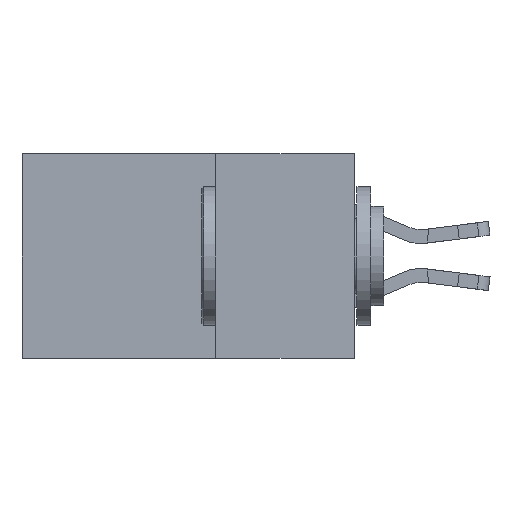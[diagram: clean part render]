
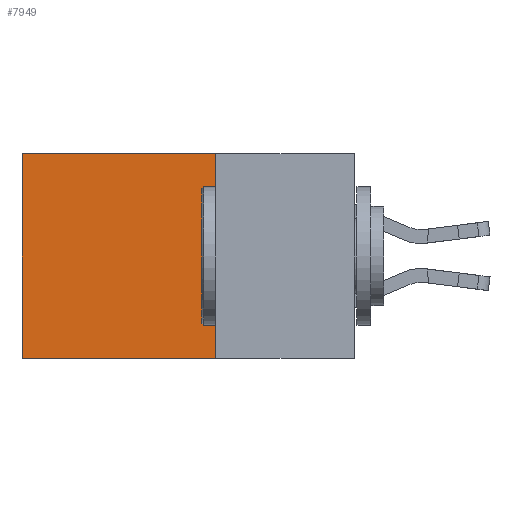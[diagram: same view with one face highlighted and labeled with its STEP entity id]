
A CAD part, left-side view. The second image highlights one B-rep face of the part: STEP entity #7949.
In plain terms, the highlighted planar face has unit normal (-1, 0, 0).
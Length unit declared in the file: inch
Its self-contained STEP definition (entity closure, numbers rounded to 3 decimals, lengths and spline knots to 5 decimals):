
#158 = DIRECTION ( 'NONE',  ( 0., 1., 0. ) ) ;
#1003 = EDGE_CURVE ( 'NONE', #11231, #4070, #4851, .T. ) ;
#1647 = ORIENTED_EDGE ( 'NONE', *, *, #11273, .F. ) ;
#1665 = VECTOR ( 'NONE', #3794, 39.37008 ) ;
#2700 = VERTEX_POINT ( 'NONE', #12612 ) ;
#3143 = VERTEX_POINT ( 'NONE', #5457 ) ;
#3479 = CARTESIAN_POINT ( 'NONE',  ( 0.2615, 0.25, -0.37 ) ) ;
#3794 = DIRECTION ( 'NONE',  ( 0., 1., 0. ) ) ;
#3870 = CARTESIAN_POINT ( 'NONE',  ( 0.2615, 0.25, 0. ) ) ;
#4070 = VERTEX_POINT ( 'NONE', #4142 ) ;
#4142 = CARTESIAN_POINT ( 'NONE',  ( 0.2615, 0.6, -0.37 ) ) ;
#4332 = LINE ( 'NONE', #3870, #1665 ) ;
#4844 = FACE_OUTER_BOUND ( 'NONE', #11598, .T. ) ;
#4851 = LINE ( 'NONE', #7050, #14524 ) ;
#4900 = CARTESIAN_POINT ( 'NONE',  ( 0.2615, 0.6, 0. ) ) ;
#5062 = DIRECTION ( 'NONE',  ( 0., 0., -1. ) ) ;
#5071 = AXIS2_PLACEMENT_3D ( 'NONE', #7172, #6859, #6843 ) ;
#5457 = CARTESIAN_POINT ( 'NONE',  ( 0.2615, 0.25, 0. ) ) ;
#6830 = VECTOR ( 'NONE', #5062, 39.37008 ) ;
#6843 = DIRECTION ( 'NONE',  ( 0., 0., -1. ) ) ;
#6859 = DIRECTION ( 'NONE',  ( 1., 0., 0. ) ) ;
#6880 = PLANE ( 'NONE',  #5071 ) ;
#7050 = CARTESIAN_POINT ( 'NONE',  ( 0.2615, 0.6, -0.37 ) ) ;
#7172 = CARTESIAN_POINT ( 'NONE',  ( 0.2615, 0.25, -0.37 ) ) ;
#7949 = ADVANCED_FACE ( 'NONE', ( #4844 ), #6880, .F. ) ;
#10195 = CARTESIAN_POINT ( 'NONE',  ( 0.2615, 0.25, -0.37 ) ) ;
#10611 = ORIENTED_EDGE ( 'NONE', *, *, #1003, .T. ) ;
#10947 = ORIENTED_EDGE ( 'NONE', *, *, #11324, .F. ) ;
#11231 = VERTEX_POINT ( 'NONE', #4900 ) ;
#11273 = EDGE_CURVE ( 'NONE', #2700, #4070, #13522, .T. ) ;
#11324 = EDGE_CURVE ( 'NONE', #3143, #2700, #12854, .T. ) ;
#11598 = EDGE_LOOP ( 'NONE', ( #10611, #1647, #10947, #13801 ) ) ;
#11751 = EDGE_CURVE ( 'NONE', #3143, #11231, #4332, .T. ) ;
#12495 = DIRECTION ( 'NONE',  ( 0., 0., -1. ) ) ;
#12612 = CARTESIAN_POINT ( 'NONE',  ( 0.2615, 0.25, -0.37 ) ) ;
#12854 = LINE ( 'NONE', #3479, #6830 ) ;
#13190 = VECTOR ( 'NONE', #158, 39.37008 ) ;
#13522 = LINE ( 'NONE', #10195, #13190 ) ;
#13801 = ORIENTED_EDGE ( 'NONE', *, *, #11751, .T. ) ;
#14524 = VECTOR ( 'NONE', #12495, 39.37008 ) ;
